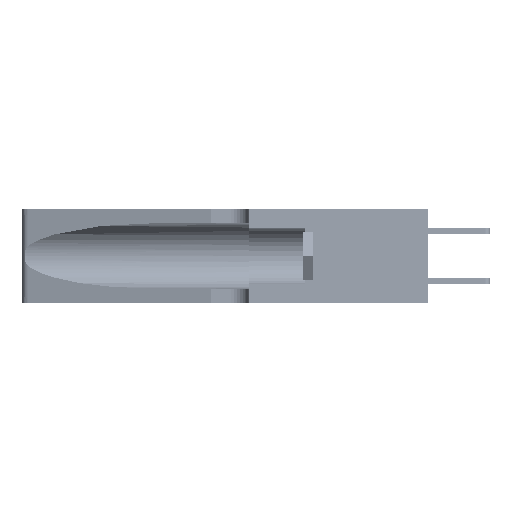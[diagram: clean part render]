
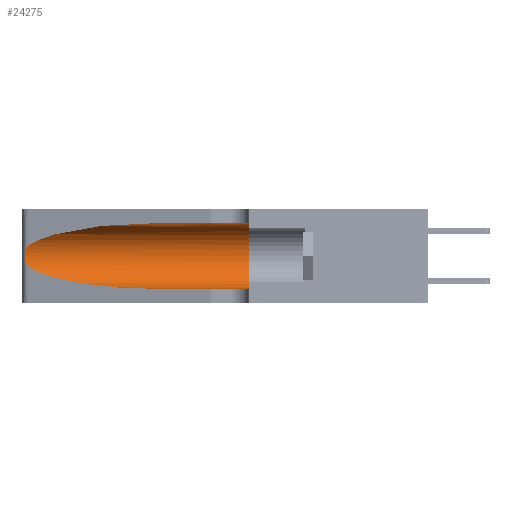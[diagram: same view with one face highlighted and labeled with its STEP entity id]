
A CAD part, left-side view. The second image highlights one B-rep face of the part: STEP entity #24275.
In plain terms, the highlighted cylindrical face has radius 3.308 mm (diameter 6.617 mm), a partial arc.
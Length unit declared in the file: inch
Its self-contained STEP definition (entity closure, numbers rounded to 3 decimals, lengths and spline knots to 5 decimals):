
#3 = CARTESIAN_POINT ( 'NONE',  ( 0.1305, 0.72297, 0.05475 ) ) ;
#1211 = CARTESIAN_POINT ( 'NONE',  ( 0.1305, 0.35, 0.05475 ) ) ;
#2186 = VERTEX_POINT ( 'NONE', #20852 ) ;
#2958 = CARTESIAN_POINT ( 'NONE',  ( 0.26075, 1.23896, 0.178 ) ) ;
#3146 = CARTESIAN_POINT ( 'NONE',  ( 0.25639, 1.23186, 0.15144 ) ) ;
#3226 = CARTESIAN_POINT ( 'NONE',  ( 0.1305, 1.61858, 0.05475 ) ) ;
#4129 = CARTESIAN_POINT ( 'NONE',  ( 0.2373, 1.15595, 0.28018 ) ) ;
#6152 = VECTOR ( 'NONE', #20414, 39.37008 ) ;
#7143 = B_SPLINE_CURVE_WITH_KNOTS ( 'NONE', 3,
 ( #28125, #23412, #19759, #40388, #19570, #15396, #35834, #2958, #19385, #14868, #36352, #3146, #52432, #15217 ),
 .UNSPECIFIED., .F., .F.,
 ( 4, 2, 2, 2, 2, 2, 4 ),
 ( 0., 0.00027, 0.00053, 0.00107, 0.0016, 0.00187, 0.00214 ),
 .UNSPECIFIED. ) ;
#7645 = CARTESIAN_POINT ( 'NONE',  ( 0.2373, 1.15595, 0.08982 ) ) ;
#8312 = EDGE_CURVE ( 'NONE', #2186, #46760, #15053, .T. ) ;
#8790 = AXIS2_PLACEMENT_3D ( 'NONE', #11786, #49339, #32926 ) ;
#9264 = VECTOR ( 'NONE', #15649, 39.37008 ) ;
#9977 = AXIS2_PLACEMENT_3D ( 'NONE', #43051, #30424, #39210 ) ;
#11313 = EDGE_LOOP ( 'NONE', ( #17458, #11756, #36873, #26812, #23556, #31267 ) ) ;
#11756 = ORIENTED_EDGE ( 'NONE', *, *, #23310, .T. ) ;
#11786 = CARTESIAN_POINT ( 'NONE',  ( 0.1305, 0.35, 0.185 ) ) ;
#11905 = LINE ( 'NONE', #3226, #9264 ) ;
#12259 = EDGE_CURVE ( 'NONE', #28053, #52737, #38633, .T. ) ;
#14868 = CARTESIAN_POINT ( 'NONE',  ( 0.25856, 1.23593, 0.16098 ) ) ;
#15053 = CIRCLE ( 'NONE', #8790, 0.13025 ) ;
#15217 = CARTESIAN_POINT ( 'NONE',  ( 0.25487, 1.22718, 0.14631 ) ) ;
#15396 = CARTESIAN_POINT ( 'NONE',  ( 0.26018, 1.23835, 0.19895 ) ) ;
#15649 = DIRECTION ( 'NONE',  ( 0., -1., 0. ) ) ;
#16052 = CARTESIAN_POINT ( 'NONE',  ( 0.1305, 0.72297, 0.05475 ) ) ;
#16236 = CARTESIAN_POINT ( 'NONE',  ( 0.25487, 1.22718, 0.22369 ) ) ;
#16367 = CARTESIAN_POINT ( 'NONE',  ( 0.25487, 1.22718, 0.22369 ) ) ;
#17458 = ORIENTED_EDGE ( 'NONE', *, *, #50524, .T. ) ;
#17891 = EDGE_CURVE ( 'NONE', #23886, #2186, #27652, .T. ) ;
#19385 = CARTESIAN_POINT ( 'NONE',  ( 0.26017, 1.23833, 0.17102 ) ) ;
#19570 = CARTESIAN_POINT ( 'NONE',  ( 0.25854, 1.2359, 0.20912 ) ) ;
#19759 = CARTESIAN_POINT ( 'NONE',  ( 0.25639, 1.23184, 0.21858 ) ) ;
#20373 = CARTESIAN_POINT ( 'NONE',  ( 0.1305, 0.72297, 0.31525 ) ) ;
#20414 = DIRECTION ( 'NONE',  ( 0., -1., 0. ) ) ;
#20852 = CARTESIAN_POINT ( 'NONE',  ( 0.1305, 0.35, 0.31525 ) ) ;
#23310 = EDGE_CURVE ( 'NONE', #33784, #28053, #7143, .T. ) ;
#23412 = CARTESIAN_POINT ( 'NONE',  ( 0.25555, 1.22994, 0.2215 ) ) ;
#23556 = ORIENTED_EDGE ( 'NONE', *, *, #8312, .F. ) ;
#23886 = VERTEX_POINT ( 'NONE', #41448 ) ;
#24237 = CARTESIAN_POINT ( 'NONE',  ( 0.1305, 1.61858, 0.31525 ) ) ;
#24249 = CARTESIAN_POINT ( 'NONE',  ( 0.25487, 1.22718, 0.14631 ) ) ;
#24275 = ADVANCED_FACE ( 'NONE', ( #26236 ), #27519, .F. ) ;
#24531 = EDGE_CURVE ( 'NONE', #52737, #46760, #11905, .T. ) ;
#26236 = FACE_OUTER_BOUND ( 'NONE', #11313, .T. ) ;
#26812 = ORIENTED_EDGE ( 'NONE', *, *, #24531, .T. ) ;
#27519 = CYLINDRICAL_SURFACE ( 'NONE', #9977, 0.13025 ) ;
#27652 = LINE ( 'NONE', #24237, #6152 ) ;
#28053 = VERTEX_POINT ( 'NONE', #30607 ) ;
#28125 = CARTESIAN_POINT ( 'NONE',  ( 0.25487, 1.22718, 0.22369 ) ) ;
#30424 = DIRECTION ( 'NONE',  ( 0., -1., 0. ) ) ;
#30607 = CARTESIAN_POINT ( 'NONE',  ( 0.25487, 1.22718, 0.14631 ) ) ;
#31267 = ORIENTED_EDGE ( 'NONE', *, *, #17891, .F. ) ;
#32926 = DIRECTION ( 'NONE',  ( 0., 0., 1. ) ) ;
#33784 = VERTEX_POINT ( 'NONE', #16236 ) ;
#35834 = CARTESIAN_POINT ( 'NONE',  ( 0.26075, 1.23896, 0.19203 ) ) ;
#36352 = CARTESIAN_POINT ( 'NONE',  ( 0.25789, 1.23486, 0.15765 ) ) ;
#36873 = ORIENTED_EDGE ( 'NONE', *, *, #12259, .T. ) ;
#37159 = CARTESIAN_POINT ( 'NONE',  ( 0.18966, 0.96281, 0.31525 ) ) ;
#38633 =( BOUNDED_CURVE ( )  B_SPLINE_CURVE ( 3, ( #24249, #7645, #41062, #16052 ),
 .UNSPECIFIED., .F., .F. ) 
 B_SPLINE_CURVE_WITH_KNOTS ( ( 4, 4 ),
 ( 3.44316, 4.71239 ),
 .UNSPECIFIED. ) 
 CURVE ( )  GEOMETRIC_REPRESENTATION_ITEM ( )  RATIONAL_B_SPLINE_CURVE ( ( 1., 0.87, 0.87, 1. ) ) 
 REPRESENTATION_ITEM ( '' )  );
#39210 = DIRECTION ( 'NONE',  ( 0., 0., -1. ) ) ;
#40388 = CARTESIAN_POINT ( 'NONE',  ( 0.25787, 1.23484, 0.2124 ) ) ;
#41062 = CARTESIAN_POINT ( 'NONE',  ( 0.18966, 0.96281, 0.05475 ) ) ;
#41448 = CARTESIAN_POINT ( 'NONE',  ( 0.1305, 0.72297, 0.31525 ) ) ;
#43051 = CARTESIAN_POINT ( 'NONE',  ( 0.1305, 1.61858, 0.185 ) ) ;
#46646 =( BOUNDED_CURVE ( )  B_SPLINE_CURVE ( 3, ( #20373, #37159, #4129, #16367 ),
 .UNSPECIFIED., .F., .F. ) 
 B_SPLINE_CURVE_WITH_KNOTS ( ( 4, 4 ),
 ( 1.5708, 2.84003 ),
 .UNSPECIFIED. ) 
 CURVE ( )  GEOMETRIC_REPRESENTATION_ITEM ( )  RATIONAL_B_SPLINE_CURVE ( ( 1., 0.87, 0.87, 1. ) ) 
 REPRESENTATION_ITEM ( '' )  );
#46760 = VERTEX_POINT ( 'NONE', #1211 ) ;
#49339 = DIRECTION ( 'NONE',  ( 0., 1., 0. ) ) ;
#50524 = EDGE_CURVE ( 'NONE', #23886, #33784, #46646, .T. ) ;
#52432 = CARTESIAN_POINT ( 'NONE',  ( 0.25555, 1.22993, 0.14849 ) ) ;
#52737 = VERTEX_POINT ( 'NONE', #3 ) ;
